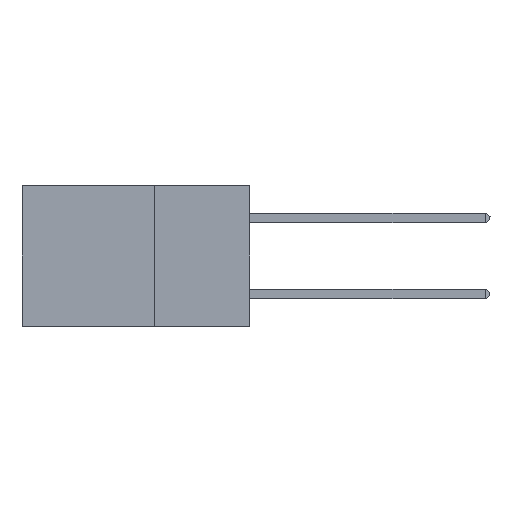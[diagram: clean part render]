
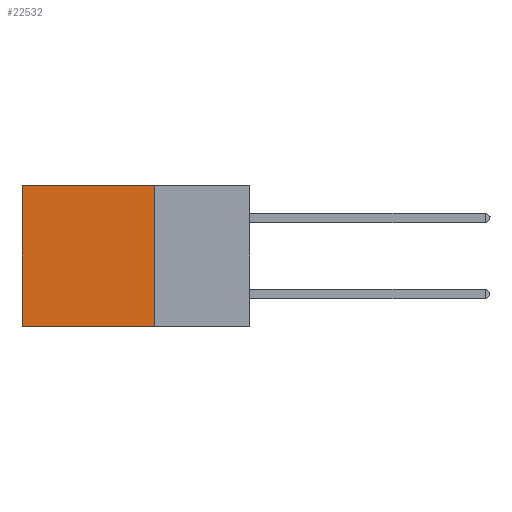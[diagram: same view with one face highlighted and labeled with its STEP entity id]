
A CAD part, left-side view. The second image highlights one B-rep face of the part: STEP entity #22532.
In plain terms, the highlighted planar face has unit normal (-1, 0, 0).
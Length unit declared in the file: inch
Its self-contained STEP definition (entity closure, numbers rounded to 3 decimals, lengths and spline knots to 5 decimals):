
#527 = VERTEX_POINT ( 'NONE', #3327 ) ;
#610 = CARTESIAN_POINT ( 'NONE',  ( 0.2875, 0.25, 0. ) ) ;
#1234 = EDGE_CURVE ( 'NONE', #527, #19811, #16860, .T. ) ;
#1481 = VECTOR ( 'NONE', #23161, 39.37008 ) ;
#2643 = DIRECTION ( 'NONE',  ( 0., 0., -1. ) ) ;
#2864 = CARTESIAN_POINT ( 'NONE',  ( 0.2875, 0.25, -0.37 ) ) ;
#3302 = CARTESIAN_POINT ( 'NONE',  ( 0.2875, 0.6, 0. ) ) ;
#3327 = CARTESIAN_POINT ( 'NONE',  ( 0.2875, 0.25, -0.37 ) ) ;
#4016 = DIRECTION ( 'NONE',  ( 0., 1., 0. ) ) ;
#4071 = EDGE_CURVE ( 'NONE', #16208, #19811, #8765, .T. ) ;
#5165 = CARTESIAN_POINT ( 'NONE',  ( 0.2875, 0.25, 0. ) ) ;
#5424 = ORIENTED_EDGE ( 'NONE', *, *, #4071, .T. ) ;
#6614 = VECTOR ( 'NONE', #19644, 39.37008 ) ;
#6654 = LINE ( 'NONE', #6765, #1481 ) ;
#6765 = CARTESIAN_POINT ( 'NONE',  ( 0.2875, 0.25, 0. ) ) ;
#7046 = VECTOR ( 'NONE', #8499, 39.37008 ) ;
#7653 = ORIENTED_EDGE ( 'NONE', *, *, #16679, .F. ) ;
#8467 = EDGE_CURVE ( 'NONE', #13989, #16208, #14368, .T. ) ;
#8499 = DIRECTION ( 'NONE',  ( 0., 1., 0. ) ) ;
#8765 = LINE ( 'NONE', #18076, #6614 ) ;
#9303 = AXIS2_PLACEMENT_3D ( 'NONE', #610, #9604, #2643 ) ;
#9604 = DIRECTION ( 'NONE',  ( 1., 0., 0. ) ) ;
#10130 = CARTESIAN_POINT ( 'NONE',  ( 0.2875, 0.6, -0.37 ) ) ;
#10728 = ORIENTED_EDGE ( 'NONE', *, *, #8467, .T. ) ;
#11504 = ORIENTED_EDGE ( 'NONE', *, *, #1234, .F. ) ;
#13989 = VERTEX_POINT ( 'NONE', #5165 ) ;
#14368 = LINE ( 'NONE', #21659, #16182 ) ;
#16173 = EDGE_LOOP ( 'NONE', ( #5424, #11504, #7653, #10728 ) ) ;
#16182 = VECTOR ( 'NONE', #4016, 39.37008 ) ;
#16208 = VERTEX_POINT ( 'NONE', #3302 ) ;
#16679 = EDGE_CURVE ( 'NONE', #13989, #527, #6654, .T. ) ;
#16860 = LINE ( 'NONE', #2864, #7046 ) ;
#18076 = CARTESIAN_POINT ( 'NONE',  ( 0.2875, 0.6, 0. ) ) ;
#18793 = PLANE ( 'NONE',  #9303 ) ;
#18928 = FACE_OUTER_BOUND ( 'NONE', #16173, .T. ) ;
#19644 = DIRECTION ( 'NONE',  ( 0., 0., -1. ) ) ;
#19811 = VERTEX_POINT ( 'NONE', #10130 ) ;
#21659 = CARTESIAN_POINT ( 'NONE',  ( 0.2875, 0.25, 0. ) ) ;
#22532 = ADVANCED_FACE ( 'NONE', ( #18928 ), #18793, .F. ) ;
#23161 = DIRECTION ( 'NONE',  ( 0., 0., -1. ) ) ;
